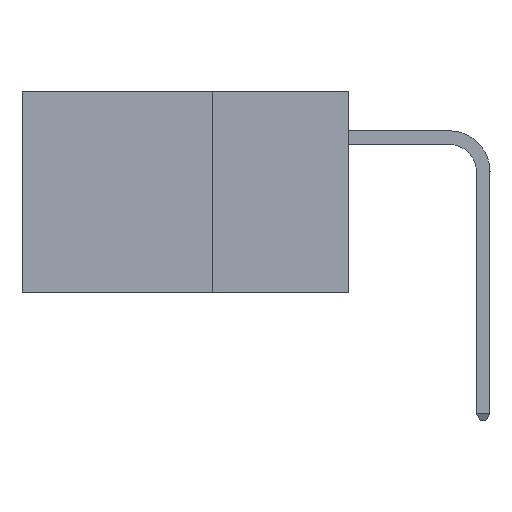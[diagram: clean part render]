
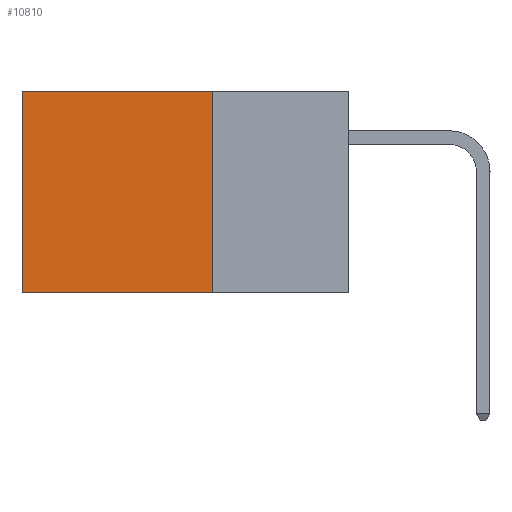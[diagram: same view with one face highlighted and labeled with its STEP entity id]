
A CAD part, left-side view. The second image highlights one B-rep face of the part: STEP entity #10810.
In plain terms, the highlighted planar face has unit normal (-1, 0, 0).
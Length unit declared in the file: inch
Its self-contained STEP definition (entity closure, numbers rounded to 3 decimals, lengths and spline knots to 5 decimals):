
#507 = CARTESIAN_POINT ( 'NONE',  ( 0.2875, 0.6, 0. ) ) ;
#812 = ORIENTED_EDGE ( 'NONE', *, *, #5979, .F. ) ;
#1136 = LINE ( 'NONE', #507, #8205 ) ;
#1515 = CARTESIAN_POINT ( 'NONE',  ( 0.2875, 0.25, 0. ) ) ;
#1602 = DIRECTION ( 'NONE',  ( 0., 0., -1. ) ) ;
#1735 = EDGE_CURVE ( 'NONE', #8317, #3674, #15234, .T. ) ;
#1855 = ORIENTED_EDGE ( 'NONE', *, *, #1735, .F. ) ;
#2033 = AXIS2_PLACEMENT_3D ( 'NONE', #10918, #12010, #4966 ) ;
#2554 = CARTESIAN_POINT ( 'NONE',  ( 0.2875, 0.6, 0. ) ) ;
#2868 = DIRECTION ( 'NONE',  ( 0., 1., 0. ) ) ;
#3273 = EDGE_LOOP ( 'NONE', ( #7142, #812, #1855, #8878 ) ) ;
#3674 = VERTEX_POINT ( 'NONE', #14685 ) ;
#3697 = PLANE ( 'NONE',  #2033 ) ;
#3957 = EDGE_CURVE ( 'NONE', #4229, #6886, #1136, .T. ) ;
#4229 = VERTEX_POINT ( 'NONE', #2554 ) ;
#4966 = DIRECTION ( 'NONE',  ( 0., 0., -1. ) ) ;
#5979 = EDGE_CURVE ( 'NONE', #3674, #6886, #6819, .T. ) ;
#6450 = VECTOR ( 'NONE', #8426, 39.37008 ) ;
#6819 = LINE ( 'NONE', #8496, #6450 ) ;
#6886 = VERTEX_POINT ( 'NONE', #13801 ) ;
#7142 = ORIENTED_EDGE ( 'NONE', *, *, #3957, .T. ) ;
#8205 = VECTOR ( 'NONE', #1602, 39.37008 ) ;
#8317 = VERTEX_POINT ( 'NONE', #11901 ) ;
#8426 = DIRECTION ( 'NONE',  ( 0., 1., 0. ) ) ;
#8496 = CARTESIAN_POINT ( 'NONE',  ( 0.2875, 0.25, -0.37 ) ) ;
#8878 = ORIENTED_EDGE ( 'NONE', *, *, #13485, .T. ) ;
#8997 = DIRECTION ( 'NONE',  ( 0., 0., -1. ) ) ;
#9156 = VECTOR ( 'NONE', #8997, 39.37008 ) ;
#9865 = LINE ( 'NONE', #1515, #15499 ) ;
#10810 = ADVANCED_FACE ( 'NONE', ( #14542 ), #3697, .F. ) ;
#10918 = CARTESIAN_POINT ( 'NONE',  ( 0.2875, 0.25, 0. ) ) ;
#11641 = CARTESIAN_POINT ( 'NONE',  ( 0.2875, 0.25, 0. ) ) ;
#11901 = CARTESIAN_POINT ( 'NONE',  ( 0.2875, 0.25, 0. ) ) ;
#12010 = DIRECTION ( 'NONE',  ( 1., 0., 0. ) ) ;
#13485 = EDGE_CURVE ( 'NONE', #8317, #4229, #9865, .T. ) ;
#13801 = CARTESIAN_POINT ( 'NONE',  ( 0.2875, 0.6, -0.37 ) ) ;
#14542 = FACE_OUTER_BOUND ( 'NONE', #3273, .T. ) ;
#14685 = CARTESIAN_POINT ( 'NONE',  ( 0.2875, 0.25, -0.37 ) ) ;
#15234 = LINE ( 'NONE', #11641, #9156 ) ;
#15499 = VECTOR ( 'NONE', #2868, 39.37008 ) ;
